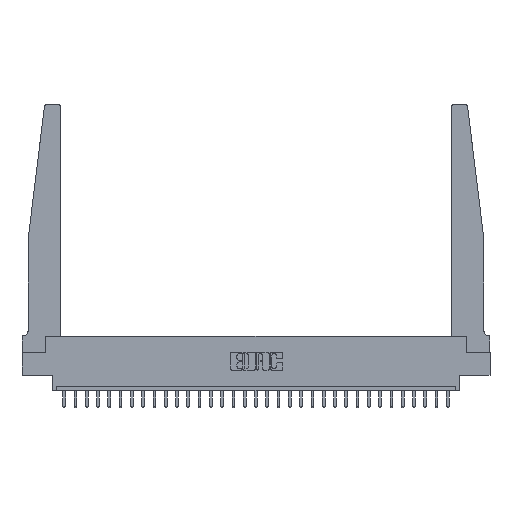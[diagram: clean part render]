
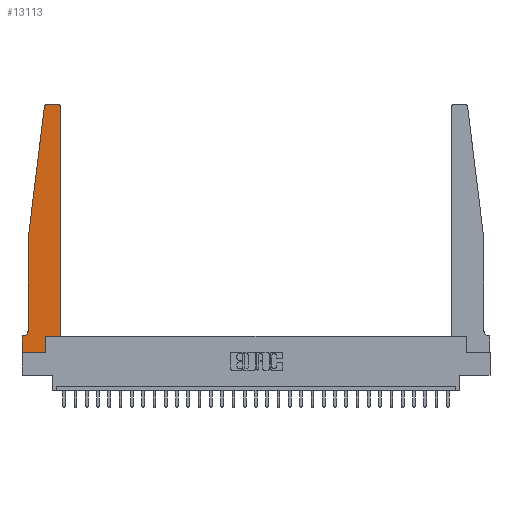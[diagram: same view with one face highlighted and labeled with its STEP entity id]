
A CAD part, top view. The second image highlights one B-rep face of the part: STEP entity #13113.
In plain terms, the highlighted planar face has unit normal (0, 0, 1).
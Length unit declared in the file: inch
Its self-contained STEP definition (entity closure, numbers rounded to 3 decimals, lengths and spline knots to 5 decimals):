
#14 = VECTOR ( 'NONE', #8791, 39.37008 ) ;
#52 = EDGE_CURVE ( 'NONE', #11474, #20823, #6726, .T. ) ;
#195 = CARTESIAN_POINT ( 'NONE',  ( 0.395, 2.72, 0.37 ) ) ;
#464 = ORIENTED_EDGE ( 'NONE', *, *, #8092, .T. ) ;
#584 = FACE_OUTER_BOUND ( 'NONE', #5559, .T. ) ;
#594 = DIRECTION ( 'NONE',  ( 0., 1., 0. ) ) ;
#835 = DIRECTION ( 'NONE',  ( -1., 0., 0. ) ) ;
#905 = CIRCLE ( 'NONE', #15907, 0.05 ) ;
#925 = EDGE_CURVE ( 'NONE', #13180, #2609, #27087, .T. ) ;
#1074 = CARTESIAN_POINT ( 'NONE',  ( 0., 0.1875, 0.37 ) ) ;
#1342 = ORIENTED_EDGE ( 'NONE', *, *, #12381, .T. ) ;
#1566 = DIRECTION ( 'NONE',  ( -1., 0., 0. ) ) ;
#1827 = CARTESIAN_POINT ( 'NONE',  ( 0.425, 2.72, 0.37 ) ) ;
#1959 = EDGE_CURVE ( 'NONE', #22217, #15993, #3689, .T. ) ;
#2609 = VERTEX_POINT ( 'NONE', #12577 ) ;
#2688 = CARTESIAN_POINT ( 'NONE',  ( 0.065, 0.2375, 0.37 ) ) ;
#2814 = CARTESIAN_POINT ( 'NONE',  ( 0.2605, 0., 0.37 ) ) ;
#2827 = VERTEX_POINT ( 'NONE', #2814 ) ;
#3215 = CARTESIAN_POINT ( 'NONE',  ( 0.065, 1.25, 0.37 ) ) ;
#3388 = DIRECTION ( 'NONE',  ( 1., 0., 0. ) ) ;
#3689 = LINE ( 'NONE', #18875, #26447 ) ;
#3736 = CARTESIAN_POINT ( 'NONE',  ( 0.27653, 2.72, 0.37 ) ) ;
#4005 = DIRECTION ( 'NONE',  ( 0., -1., 0. ) ) ;
#4151 = ORIENTED_EDGE ( 'NONE', *, *, #13965, .T. ) ;
#4390 = DIRECTION ( 'NONE',  ( 1., 0., 0. ) ) ;
#4472 = CARTESIAN_POINT ( 'NONE',  ( 0.425, 0.18, 0.37 ) ) ;
#5032 = CARTESIAN_POINT ( 'NONE',  ( 0.395, 2.75, 0.37 ) ) ;
#5383 = AXIS2_PLACEMENT_3D ( 'NONE', #1074, #11958, #3388 ) ;
#5428 = CARTESIAN_POINT ( 'NONE',  ( 0.065, 1.25, 0.37 ) ) ;
#5559 = EDGE_LOOP ( 'NONE', ( #12374, #26638, #5850, #11526, #1342, #13981, #464, #13380, #24200, #25388, #4151, #22876 ) ) ;
#5850 = ORIENTED_EDGE ( 'NONE', *, *, #16234, .T. ) ;
#6196 = EDGE_CURVE ( 'NONE', #6662, #2827, #24227, .T. ) ;
#6662 = VERTEX_POINT ( 'NONE', #7251 ) ;
#6726 = LINE ( 'NONE', #27368, #15374 ) ;
#7251 = CARTESIAN_POINT ( 'NONE',  ( 0., 0., 0.37 ) ) ;
#7262 = DIRECTION ( 'NONE',  ( 0., 1., 0. ) ) ;
#7874 = AXIS2_PLACEMENT_3D ( 'NONE', #195, #10799, #21457 ) ;
#8087 = VERTEX_POINT ( 'NONE', #1827 ) ;
#8092 = EDGE_CURVE ( 'NONE', #2609, #6662, #10105, .T. ) ;
#8791 = DIRECTION ( 'NONE',  ( -1., 0., 0. ) ) ;
#9055 = VERTEX_POINT ( 'NONE', #12289 ) ;
#9173 = VECTOR ( 'NONE', #7262, 39.37008 ) ;
#10105 = LINE ( 'NONE', #27068, #18120 ) ;
#10174 = VECTOR ( 'NONE', #594, 39.37008 ) ;
#10348 = EDGE_CURVE ( 'NONE', #15993, #27024, #11999, .T. ) ;
#10799 = DIRECTION ( 'NONE',  ( 0., 0., 1. ) ) ;
#11474 = VERTEX_POINT ( 'NONE', #5428 ) ;
#11526 = ORIENTED_EDGE ( 'NONE', *, *, #52, .T. ) ;
#11958 = DIRECTION ( 'NONE',  ( 0., 0., 1. ) ) ;
#11999 = CIRCLE ( 'NONE', #26849, 0.03 ) ;
#12289 = CARTESIAN_POINT ( 'NONE',  ( 0.2605, 0.18, 0.37 ) ) ;
#12374 = ORIENTED_EDGE ( 'NONE', *, *, #1959, .T. ) ;
#12381 = EDGE_CURVE ( 'NONE', #20823, #13180, #905, .T. ) ;
#12577 = CARTESIAN_POINT ( 'NONE',  ( 0., 0.1875, 0.37 ) ) ;
#12587 = CIRCLE ( 'NONE', #7874, 0.03 ) ;
#12915 = CARTESIAN_POINT ( 'NONE',  ( 0.065, 0.1875, 0.37 ) ) ;
#13113 = ADVANCED_FACE ( 'NONE', ( #584 ), #22622, .T. ) ;
#13180 = VERTEX_POINT ( 'NONE', #14358 ) ;
#13380 = ORIENTED_EDGE ( 'NONE', *, *, #6196, .T. ) ;
#13531 = LINE ( 'NONE', #15652, #9173 ) ;
#13917 = DIRECTION ( 'NONE',  ( 1., 0., 0. ) ) ;
#13923 = CARTESIAN_POINT ( 'NONE',  ( 0.24675, 2.72367, 0.37 ) ) ;
#13965 = EDGE_CURVE ( 'NONE', #24871, #8087, #22240, .T. ) ;
#13981 = ORIENTED_EDGE ( 'NONE', *, *, #925, .T. ) ;
#14197 = DIRECTION ( 'NONE',  ( 0., -1., 0. ) ) ;
#14358 = CARTESIAN_POINT ( 'NONE',  ( 0.015, 0.1875, 0.37 ) ) ;
#14402 = EDGE_CURVE ( 'NONE', #9055, #24871, #25193, .T. ) ;
#14606 = DIRECTION ( 'NONE',  ( 0., 0., 1. ) ) ;
#15374 = VECTOR ( 'NONE', #4005, 39.37008 ) ;
#15652 = CARTESIAN_POINT ( 'NONE',  ( 0.2605, 0.18, 0.37 ) ) ;
#15715 = CARTESIAN_POINT ( 'NONE',  ( 0.015, 0.2375, 0.37 ) ) ;
#15907 = AXIS2_PLACEMENT_3D ( 'NONE', #15715, #17587, #835 ) ;
#15993 = VERTEX_POINT ( 'NONE', #16504 ) ;
#16234 = EDGE_CURVE ( 'NONE', #27024, #11474, #17689, .T. ) ;
#16347 = VECTOR ( 'NONE', #26499, 39.37008 ) ;
#16504 = CARTESIAN_POINT ( 'NONE',  ( 0.27653, 2.75, 0.37 ) ) ;
#17525 = CARTESIAN_POINT ( 'NONE',  ( 0.425, 0.18, 0.37 ) ) ;
#17587 = DIRECTION ( 'NONE',  ( 0., 0., -1. ) ) ;
#17689 = LINE ( 'NONE', #3215, #16347 ) ;
#18120 = VECTOR ( 'NONE', #14197, 39.37008 ) ;
#18875 = CARTESIAN_POINT ( 'NONE',  ( 0.25, 2.75, 0.37 ) ) ;
#18900 = DIRECTION ( 'NONE',  ( 1., 0., 0. ) ) ;
#19140 = VECTOR ( 'NONE', #13917, 39.37008 ) ;
#20823 = VERTEX_POINT ( 'NONE', #2688 ) ;
#21457 = DIRECTION ( 'NONE',  ( 1., 0., 0. ) ) ;
#22217 = VERTEX_POINT ( 'NONE', #5032 ) ;
#22240 = LINE ( 'NONE', #24020, #10174 ) ;
#22622 = PLANE ( 'NONE',  #5383 ) ;
#22876 = ORIENTED_EDGE ( 'NONE', *, *, #24015, .T. ) ;
#24015 = EDGE_CURVE ( 'NONE', #8087, #22217, #12587, .T. ) ;
#24020 = CARTESIAN_POINT ( 'NONE',  ( 0.425, 0.18, 0.37 ) ) ;
#24200 = ORIENTED_EDGE ( 'NONE', *, *, #25055, .T. ) ;
#24227 = LINE ( 'NONE', #26777, #19140 ) ;
#24871 = VERTEX_POINT ( 'NONE', #17525 ) ;
#25055 = EDGE_CURVE ( 'NONE', #2827, #9055, #13531, .T. ) ;
#25193 = LINE ( 'NONE', #4472, #25889 ) ;
#25388 = ORIENTED_EDGE ( 'NONE', *, *, #14402, .T. ) ;
#25889 = VECTOR ( 'NONE', #4390, 39.37008 ) ;
#26447 = VECTOR ( 'NONE', #1566, 39.37008 ) ;
#26499 = DIRECTION ( 'NONE',  ( -0.122, -0.992, 0. ) ) ;
#26638 = ORIENTED_EDGE ( 'NONE', *, *, #10348, .T. ) ;
#26777 = CARTESIAN_POINT ( 'NONE',  ( 0., 0., 0.37 ) ) ;
#26849 = AXIS2_PLACEMENT_3D ( 'NONE', #3736, #14606, #18900 ) ;
#27024 = VERTEX_POINT ( 'NONE', #13923 ) ;
#27068 = CARTESIAN_POINT ( 'NONE',  ( 0., 0., 0.37 ) ) ;
#27087 = LINE ( 'NONE', #12915, #14 ) ;
#27368 = CARTESIAN_POINT ( 'NONE',  ( 0.065, 1.25, 0.37 ) ) ;
